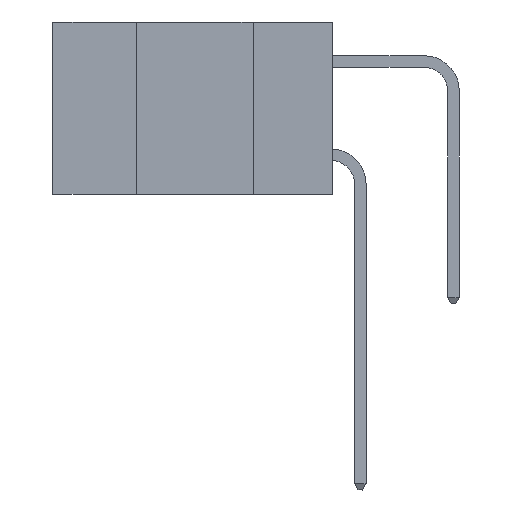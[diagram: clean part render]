
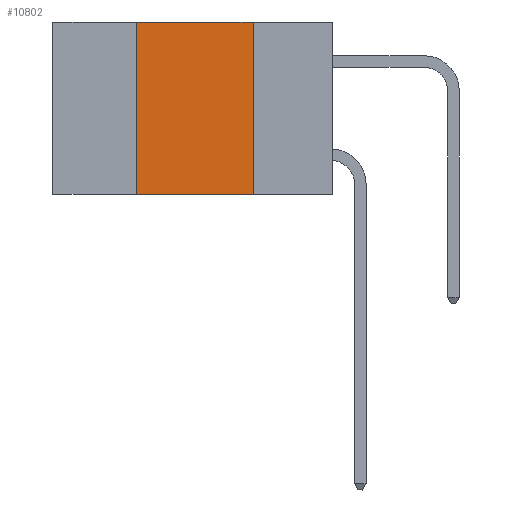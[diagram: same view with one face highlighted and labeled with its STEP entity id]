
A CAD part, left-side view. The second image highlights one B-rep face of the part: STEP entity #10802.
In plain terms, the highlighted planar face has unit normal (-1, 0, 0).
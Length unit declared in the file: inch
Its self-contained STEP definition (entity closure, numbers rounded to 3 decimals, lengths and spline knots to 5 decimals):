
#407 = LINE ( 'NONE', #18200, #29004 ) ;
#483 = VECTOR ( 'NONE', #24053, 39.37008 ) ;
#539 = EDGE_CURVE ( 'NONE', #5594, #19862, #23811, .T. ) ;
#687 = ORIENTED_EDGE ( 'NONE', *, *, #13140, .F. ) ;
#1516 = DIRECTION ( 'NONE',  ( 0., 0., -1. ) ) ;
#3276 = CARTESIAN_POINT ( 'NONE',  ( 0., 0.42, -0.37 ) ) ;
#3352 = EDGE_CURVE ( 'NONE', #5594, #10666, #407, .T. ) ;
#3585 = CARTESIAN_POINT ( 'NONE',  ( 0., 0.17, -0.37 ) ) ;
#5594 = VERTEX_POINT ( 'NONE', #3276 ) ;
#5824 = LINE ( 'NONE', #13266, #11166 ) ;
#6981 = CARTESIAN_POINT ( 'NONE',  ( 0., 0.17, 0. ) ) ;
#10666 = VERTEX_POINT ( 'NONE', #12192 ) ;
#10802 = ADVANCED_FACE ( 'NONE', ( #20823 ), #28565, .F. ) ;
#11166 = VECTOR ( 'NONE', #24520, 39.37008 ) ;
#12192 = CARTESIAN_POINT ( 'NONE',  ( 0., 0.42, 0. ) ) ;
#12709 = ORIENTED_EDGE ( 'NONE', *, *, #3352, .F. ) ;
#12885 = VERTEX_POINT ( 'NONE', #19169 ) ;
#13140 = EDGE_CURVE ( 'NONE', #10666, #12885, #5824, .T. ) ;
#13266 = CARTESIAN_POINT ( 'NONE',  ( 0., 0.6, 0. ) ) ;
#13292 = AXIS2_PLACEMENT_3D ( 'NONE', #26197, #15052, #1516 ) ;
#13955 = EDGE_CURVE ( 'NONE', #12885, #19862, #16316, .T. ) ;
#15052 = DIRECTION ( 'NONE',  ( 1., 0., 0. ) ) ;
#15631 = VECTOR ( 'NONE', #20498, 39.37008 ) ;
#16316 = LINE ( 'NONE', #6981, #15631 ) ;
#17966 = ORIENTED_EDGE ( 'NONE', *, *, #13955, .F. ) ;
#18200 = CARTESIAN_POINT ( 'NONE',  ( 0., 0.42, 0. ) ) ;
#19169 = CARTESIAN_POINT ( 'NONE',  ( 0., 0.17, 0. ) ) ;
#19862 = VERTEX_POINT ( 'NONE', #3585 ) ;
#20498 = DIRECTION ( 'NONE',  ( 0., 0., -1. ) ) ;
#20582 = DIRECTION ( 'NONE',  ( 0., 0., 1. ) ) ;
#20823 = FACE_OUTER_BOUND ( 'NONE', #29199, .T. ) ;
#23811 = LINE ( 'NONE', #28285, #483 ) ;
#24053 = DIRECTION ( 'NONE',  ( 0., -1., 0. ) ) ;
#24520 = DIRECTION ( 'NONE',  ( 0., -1., 0. ) ) ;
#25403 = ORIENTED_EDGE ( 'NONE', *, *, #539, .T. ) ;
#26197 = CARTESIAN_POINT ( 'NONE',  ( 0., 0.6, 0. ) ) ;
#28285 = CARTESIAN_POINT ( 'NONE',  ( 0., 0.6, -0.37 ) ) ;
#28565 = PLANE ( 'NONE',  #13292 ) ;
#29004 = VECTOR ( 'NONE', #20582, 39.37008 ) ;
#29199 = EDGE_LOOP ( 'NONE', ( #17966, #687, #12709, #25403 ) ) ;
